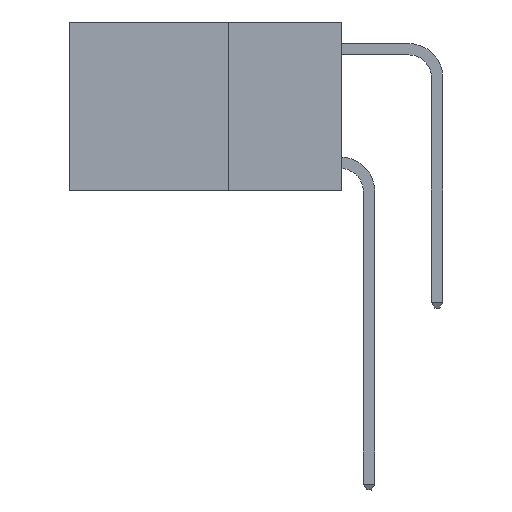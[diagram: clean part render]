
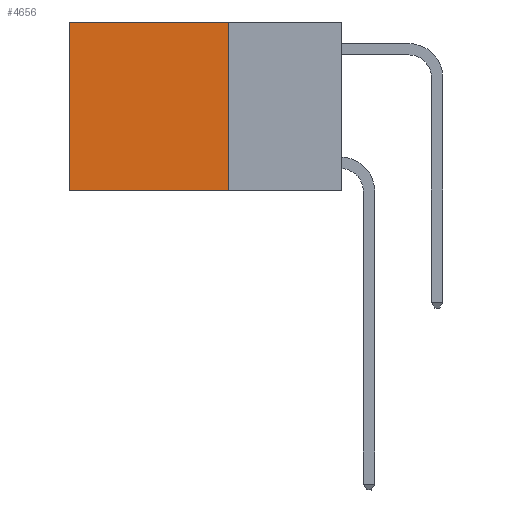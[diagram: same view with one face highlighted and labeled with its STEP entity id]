
A CAD part, left-side view. The second image highlights one B-rep face of the part: STEP entity #4656.
In plain terms, the highlighted planar face has unit normal (-1, 0, 0).
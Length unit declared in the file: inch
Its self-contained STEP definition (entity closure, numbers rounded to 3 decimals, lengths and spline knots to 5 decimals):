
#124 = CARTESIAN_POINT ( 'NONE',  ( 0.2625, 0.6, 0. ) ) ;
#1050 = CARTESIAN_POINT ( 'NONE',  ( 0.2625, 0.6, -0.37 ) ) ;
#1100 = ORIENTED_EDGE ( 'NONE', *, *, #10902, .T. ) ;
#1147 = FACE_OUTER_BOUND ( 'NONE', #14567, .T. ) ;
#1293 = LINE ( 'NONE', #2887, #4581 ) ;
#1351 = CARTESIAN_POINT ( 'NONE',  ( 0.2625, 0.25, 0. ) ) ;
#1985 = CARTESIAN_POINT ( 'NONE',  ( 0.2625, 0.25, -0.37 ) ) ;
#2138 = VECTOR ( 'NONE', #11465, 39.37008 ) ;
#2626 = PLANE ( 'NONE',  #13172 ) ;
#2710 = CARTESIAN_POINT ( 'NONE',  ( 0.2625, 0.6, 0. ) ) ;
#2887 = CARTESIAN_POINT ( 'NONE',  ( 0.2625, 0.25, 0. ) ) ;
#2942 = LINE ( 'NONE', #1985, #2138 ) ;
#3652 = ORIENTED_EDGE ( 'NONE', *, *, #9057, .F. ) ;
#3818 = VECTOR ( 'NONE', #3945, 39.37008 ) ;
#3867 = DIRECTION ( 'NONE',  ( 0., 0., -1. ) ) ;
#3945 = DIRECTION ( 'NONE',  ( 0., 0., -1. ) ) ;
#4581 = VECTOR ( 'NONE', #14575, 39.37008 ) ;
#4656 = ADVANCED_FACE ( 'NONE', ( #1147 ), #2626, .F. ) ;
#5170 = CARTESIAN_POINT ( 'NONE',  ( 0.2625, 0.25, -0.37 ) ) ;
#5278 = VERTEX_POINT ( 'NONE', #6158 ) ;
#6158 = CARTESIAN_POINT ( 'NONE',  ( 0.2625, 0.25, 0. ) ) ;
#6163 = DIRECTION ( 'NONE',  ( 0., 0., -1. ) ) ;
#7342 = DIRECTION ( 'NONE',  ( 1., 0., 0. ) ) ;
#7702 = VERTEX_POINT ( 'NONE', #5170 ) ;
#7964 = VECTOR ( 'NONE', #6163, 39.37008 ) ;
#9057 = EDGE_CURVE ( 'NONE', #7702, #12840, #2942, .T. ) ;
#10051 = LINE ( 'NONE', #2710, #3818 ) ;
#10122 = ORIENTED_EDGE ( 'NONE', *, *, #14152, .F. ) ;
#10704 = LINE ( 'NONE', #13168, #7964 ) ;
#10902 = EDGE_CURVE ( 'NONE', #5278, #11412, #1293, .T. ) ;
#11412 = VERTEX_POINT ( 'NONE', #124 ) ;
#11449 = EDGE_CURVE ( 'NONE', #11412, #12840, #10051, .T. ) ;
#11465 = DIRECTION ( 'NONE',  ( 0., 1., 0. ) ) ;
#12840 = VERTEX_POINT ( 'NONE', #1050 ) ;
#13168 = CARTESIAN_POINT ( 'NONE',  ( 0.2625, 0.25, 0. ) ) ;
#13172 = AXIS2_PLACEMENT_3D ( 'NONE', #1351, #7342, #3867 ) ;
#14031 = ORIENTED_EDGE ( 'NONE', *, *, #11449, .T. ) ;
#14152 = EDGE_CURVE ( 'NONE', #5278, #7702, #10704, .T. ) ;
#14567 = EDGE_LOOP ( 'NONE', ( #14031, #3652, #10122, #1100 ) ) ;
#14575 = DIRECTION ( 'NONE',  ( 0., 1., 0. ) ) ;
